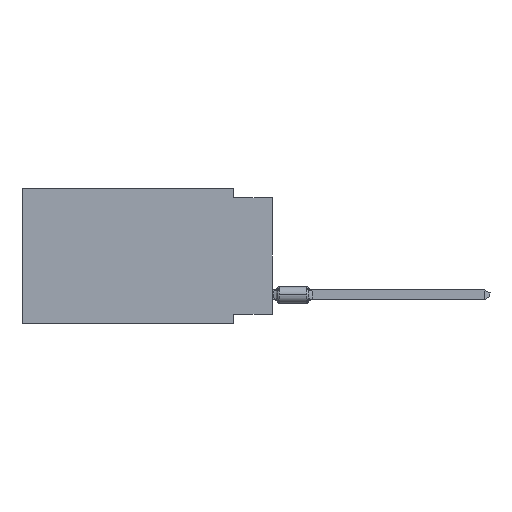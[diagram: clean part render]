
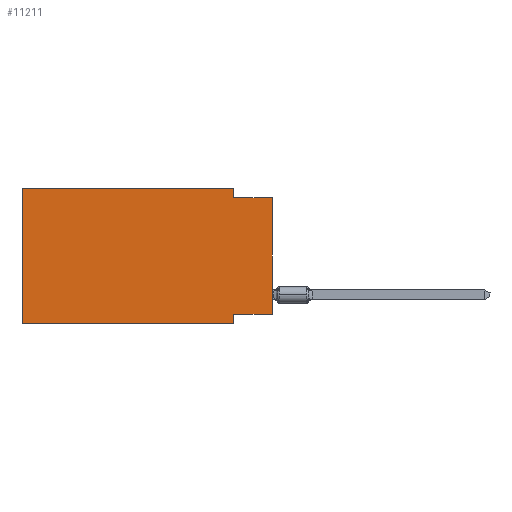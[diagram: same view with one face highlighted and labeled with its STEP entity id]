
A CAD part, left-side view. The second image highlights one B-rep face of the part: STEP entity #11211.
In plain terms, the highlighted planar face has unit normal (-1, 0, 0).
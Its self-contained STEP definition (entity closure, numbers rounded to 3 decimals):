
#87 = CARTESIAN_POINT ( 'NONE',  ( 0., 0., -8.255 ) ) ;
#711 = VECTOR ( 'NONE', #33138, 1000. ) ;
#1288 = PLANE ( 'NONE',  #23768 ) ;
#2088 = CARTESIAN_POINT ( 'NONE',  ( 0., 16.383, 0. ) ) ;
#3122 = EDGE_CURVE ( 'NONE', #28502, #27784, #11671, .T. ) ;
#3147 = VERTEX_POINT ( 'NONE', #4145 ) ;
#4145 = CARTESIAN_POINT ( 'NONE',  ( 0., 2.54, -8.255 ) ) ;
#4588 = LINE ( 'NONE', #17673, #8460 ) ;
#5514 = DIRECTION ( 'NONE',  ( 0., 1., 0. ) ) ;
#5624 = CARTESIAN_POINT ( 'NONE',  ( 0., 16.383, 0. ) ) ;
#6024 = EDGE_CURVE ( 'NONE', #10802, #3147, #28891, .T. ) ;
#6519 = VECTOR ( 'NONE', #26999, 1000. ) ;
#7011 = ORIENTED_EDGE ( 'NONE', *, *, #29887, .F. ) ;
#8460 = VECTOR ( 'NONE', #34080, 1000. ) ;
#8652 = VECTOR ( 'NONE', #27885, 1000. ) ;
#9505 = EDGE_LOOP ( 'NONE', ( #12623, #19864, #12986, #30095, #7011, #33933, #30160, #10281 ) ) ;
#10281 = ORIENTED_EDGE ( 'NONE', *, *, #6024, .F. ) ;
#10566 = VECTOR ( 'NONE', #22477, 1000. ) ;
#10592 = VERTEX_POINT ( 'NONE', #2088 ) ;
#10622 = CARTESIAN_POINT ( 'NONE',  ( 0., 16.383, 0. ) ) ;
#10802 = VERTEX_POINT ( 'NONE', #18667 ) ;
#11211 = ADVANCED_FACE ( 'NONE', ( #19626 ), #1288, .F. ) ;
#11307 = CARTESIAN_POINT ( 'NONE',  ( 0., 2.54, 0. ) ) ;
#11423 = CARTESIAN_POINT ( 'NONE',  ( 0., 16.383, 0. ) ) ;
#11482 = CARTESIAN_POINT ( 'NONE',  ( 0., 0., -0.635 ) ) ;
#11671 = LINE ( 'NONE', #11482, #10566 ) ;
#11709 = CARTESIAN_POINT ( 'NONE',  ( 0., 16.383, -8.89 ) ) ;
#12623 = ORIENTED_EDGE ( 'NONE', *, *, #27335, .T. ) ;
#12986 = ORIENTED_EDGE ( 'NONE', *, *, #15784, .F. ) ;
#13045 = DIRECTION ( 'NONE',  ( 0., 0., 1. ) ) ;
#13293 = DIRECTION ( 'NONE',  ( 0., 0., 1. ) ) ;
#14117 = CARTESIAN_POINT ( 'NONE',  ( 0., 2.54, 0. ) ) ;
#14974 = EDGE_CURVE ( 'NONE', #31818, #31561, #4588, .T. ) ;
#15154 = CARTESIAN_POINT ( 'NONE',  ( 0., 0., 0. ) ) ;
#15196 = CARTESIAN_POINT ( 'NONE',  ( 0., 2.54, -8.89 ) ) ;
#15315 = LINE ( 'NONE', #15154, #27920 ) ;
#15784 = EDGE_CURVE ( 'NONE', #23643, #28502, #22148, .T. ) ;
#16533 = LINE ( 'NONE', #30326, #8652 ) ;
#17673 = CARTESIAN_POINT ( 'NONE',  ( 0., 16.383, -8.89 ) ) ;
#17891 = VECTOR ( 'NONE', #13293, 1000. ) ;
#18667 = CARTESIAN_POINT ( 'NONE',  ( 0., 0., -8.255 ) ) ;
#18882 = LINE ( 'NONE', #5624, #17891 ) ;
#18942 = EDGE_CURVE ( 'NONE', #3147, #31561, #16533, .T. ) ;
#19122 = CARTESIAN_POINT ( 'NONE',  ( 0., 0., -0.635 ) ) ;
#19626 = FACE_OUTER_BOUND ( 'NONE', #9505, .T. ) ;
#19864 = ORIENTED_EDGE ( 'NONE', *, *, #3122, .F. ) ;
#21254 = LINE ( 'NONE', #10622, #6519 ) ;
#22148 = LINE ( 'NONE', #14117, #711 ) ;
#22251 = DIRECTION ( 'NONE',  ( 1., 0., 0. ) ) ;
#22477 = DIRECTION ( 'NONE',  ( 0., -1., 0. ) ) ;
#22582 = DIRECTION ( 'NONE',  ( 0., 0., -1. ) ) ;
#23643 = VERTEX_POINT ( 'NONE', #11307 ) ;
#23768 = AXIS2_PLACEMENT_3D ( 'NONE', #11423, #22251, #22582 ) ;
#25319 = CARTESIAN_POINT ( 'NONE',  ( 0., 2.54, -0.635 ) ) ;
#26084 = VECTOR ( 'NONE', #5514, 1000. ) ;
#26999 = DIRECTION ( 'NONE',  ( 0., -1., 0. ) ) ;
#27335 = EDGE_CURVE ( 'NONE', #10802, #27784, #15315, .T. ) ;
#27784 = VERTEX_POINT ( 'NONE', #19122 ) ;
#27885 = DIRECTION ( 'NONE',  ( 0., 0., -1. ) ) ;
#27920 = VECTOR ( 'NONE', #13045, 1000. ) ;
#28502 = VERTEX_POINT ( 'NONE', #25319 ) ;
#28891 = LINE ( 'NONE', #87, #26084 ) ;
#29887 = EDGE_CURVE ( 'NONE', #31818, #10592, #18882, .T. ) ;
#30095 = ORIENTED_EDGE ( 'NONE', *, *, #32050, .F. ) ;
#30160 = ORIENTED_EDGE ( 'NONE', *, *, #18942, .F. ) ;
#30326 = CARTESIAN_POINT ( 'NONE',  ( 0., 2.54, -8.89 ) ) ;
#31561 = VERTEX_POINT ( 'NONE', #15196 ) ;
#31818 = VERTEX_POINT ( 'NONE', #11709 ) ;
#32050 = EDGE_CURVE ( 'NONE', #10592, #23643, #21254, .T. ) ;
#33138 = DIRECTION ( 'NONE',  ( 0., 0., -1. ) ) ;
#33933 = ORIENTED_EDGE ( 'NONE', *, *, #14974, .T. ) ;
#34080 = DIRECTION ( 'NONE',  ( 0., -1., 0. ) ) ;
